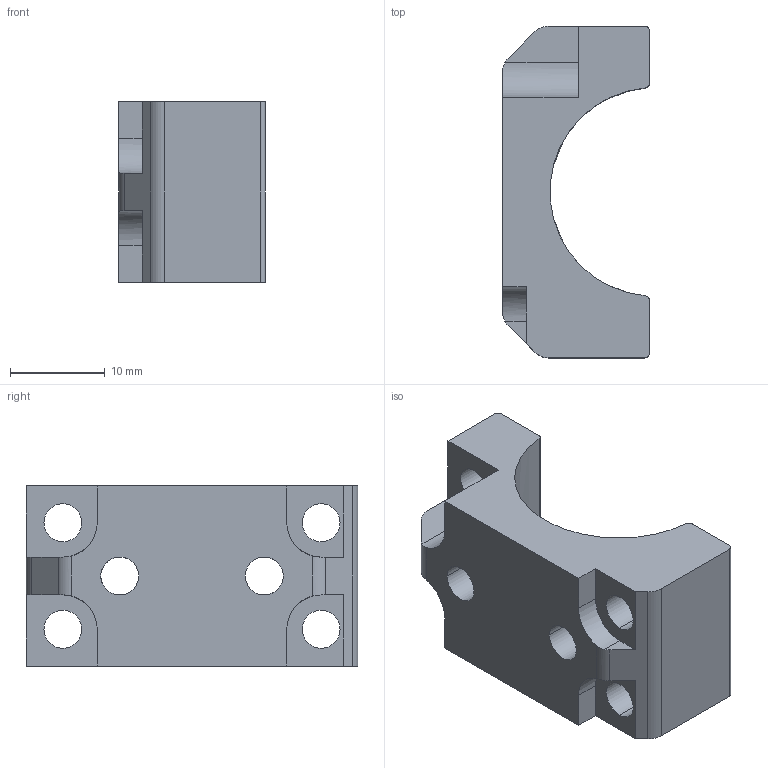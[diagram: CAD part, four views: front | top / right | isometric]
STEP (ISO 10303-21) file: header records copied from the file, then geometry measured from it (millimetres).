
FILE_DESCRIPTION (( 'STEP AP203' ), '1' );
FILE_NAME ('FREE FLOAT CLAMSHELL.STEP', '2020-10-17T20:19:28', ( '' ), ( '' ), 'SwSTEP 2.0', 'SolidWorks 2014', '' );
FILE_SCHEMA (( 'CONFIG_CONTROL_DESIGN' ));
Length unit declared in the file: millimetre
Products named in the file (2): FREE FLOAT CLAMSHELL
Bounding box: 15.5 x 35 x 19 mm (x, y, z)
Volume: 4974.5 mm3; surface area: 3313.3 mm2
Topology: 1 solids, 1 shells, 46 faces, 132 edges, 88 vertices
Faces by surface type: cylinder 25, plane 21
Entity records: 1809 total; most frequent: CARTESIAN_POINT 392, DIRECTION 266, ORIENTED_EDGE 264, EDGE_CURVE 132, AXIS2_PLACEMENT_3D 94, VERTEX_POINT 88, VECTOR 78, LINE 78
